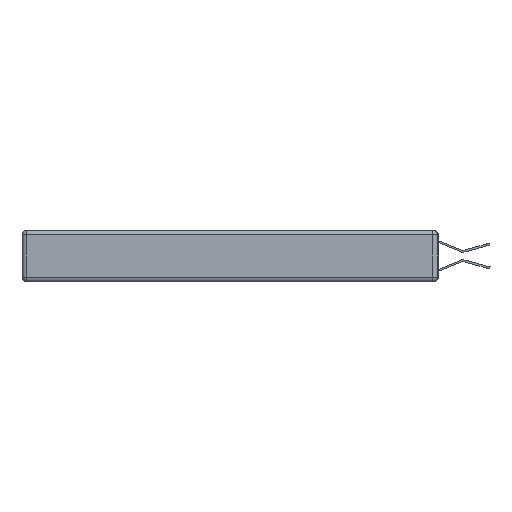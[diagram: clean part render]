
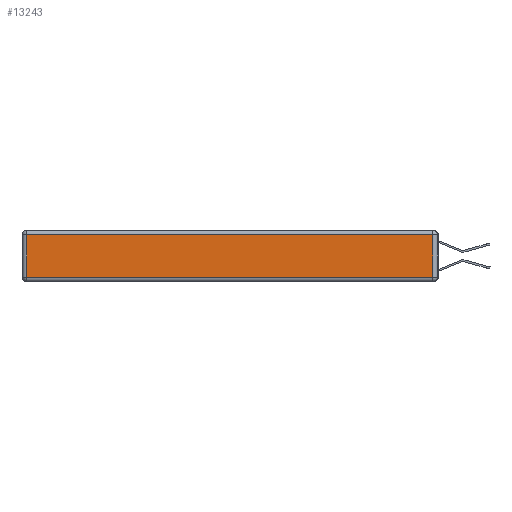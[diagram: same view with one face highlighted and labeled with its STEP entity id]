
A CAD part, left-side view. The second image highlights one B-rep face of the part: STEP entity #13243.
In plain terms, the highlighted planar face has unit normal (-1, 0, 0).
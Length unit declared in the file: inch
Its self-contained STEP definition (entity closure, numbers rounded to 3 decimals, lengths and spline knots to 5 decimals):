
#1294 = DIRECTION ( 'NONE',  ( 0., -1., 0. ) ) ;
#1480 = CARTESIAN_POINT ( 'NONE',  ( 0., 0., -0.313 ) ) ;
#1613 = DIRECTION ( 'NONE',  ( 0., 0., 1. ) ) ;
#2036 = EDGE_CURVE ( 'NONE', #18540, #14496, #18934, .T. ) ;
#2972 = DIRECTION ( 'NONE',  ( 0., 0., 1. ) ) ;
#3874 = FACE_OUTER_BOUND ( 'NONE', #13754, .T. ) ;
#4489 = ORIENTED_EDGE ( 'NONE', *, *, #10405, .T. ) ;
#5695 = EDGE_CURVE ( 'NONE', #16577, #18540, #15869, .T. ) ;
#6025 = CARTESIAN_POINT ( 'NONE',  ( 0., 0.03, -0.03 ) ) ;
#6192 = PLANE ( 'NONE',  #6915 ) ;
#6381 = CARTESIAN_POINT ( 'NONE',  ( 0., 0., -0.343 ) ) ;
#6915 = AXIS2_PLACEMENT_3D ( 'NONE', #6381, #13759, #1613 ) ;
#8147 = CARTESIAN_POINT ( 'NONE',  ( 0., 2.72, -0.03 ) ) ;
#9110 = LINE ( 'NONE', #17130, #9327 ) ;
#9327 = VECTOR ( 'NONE', #16999, 39.37008 ) ;
#9765 = VECTOR ( 'NONE', #11038, 39.37008 ) ;
#10162 = ORIENTED_EDGE ( 'NONE', *, *, #2036, .T. ) ;
#10405 = EDGE_CURVE ( 'NONE', #11205, #16577, #9110, .T. ) ;
#11038 = DIRECTION ( 'NONE',  ( 0., 1., 0. ) ) ;
#11205 = VERTEX_POINT ( 'NONE', #8147 ) ;
#11363 = CARTESIAN_POINT ( 'NONE',  ( 0., 0.03, -0.313 ) ) ;
#12005 = ORIENTED_EDGE ( 'NONE', *, *, #5695, .T. ) ;
#13243 = ADVANCED_FACE ( 'NONE', ( #3874 ), #6192, .T. ) ;
#13754 = EDGE_LOOP ( 'NONE', ( #12005, #10162, #13986, #4489 ) ) ;
#13759 = DIRECTION ( 'NONE',  ( -1., 0., 0. ) ) ;
#13986 = ORIENTED_EDGE ( 'NONE', *, *, #18415, .T. ) ;
#14193 = VECTOR ( 'NONE', #1294, 39.37008 ) ;
#14496 = VERTEX_POINT ( 'NONE', #6025 ) ;
#14809 = CARTESIAN_POINT ( 'NONE',  ( 0., 0.03, -0.343 ) ) ;
#15220 = CARTESIAN_POINT ( 'NONE',  ( 0., 2.72, -0.313 ) ) ;
#15474 = CARTESIAN_POINT ( 'NONE',  ( 0., 2.75, -0.03 ) ) ;
#15869 = LINE ( 'NONE', #1480, #14193 ) ;
#16577 = VERTEX_POINT ( 'NONE', #15220 ) ;
#16999 = DIRECTION ( 'NONE',  ( 0., 0., -1. ) ) ;
#17130 = CARTESIAN_POINT ( 'NONE',  ( 0., 2.72, -0.343 ) ) ;
#17791 = LINE ( 'NONE', #15474, #9765 ) ;
#18013 = VECTOR ( 'NONE', #2972, 39.37008 ) ;
#18415 = EDGE_CURVE ( 'NONE', #14496, #11205, #17791, .T. ) ;
#18540 = VERTEX_POINT ( 'NONE', #11363 ) ;
#18934 = LINE ( 'NONE', #14809, #18013 ) ;
